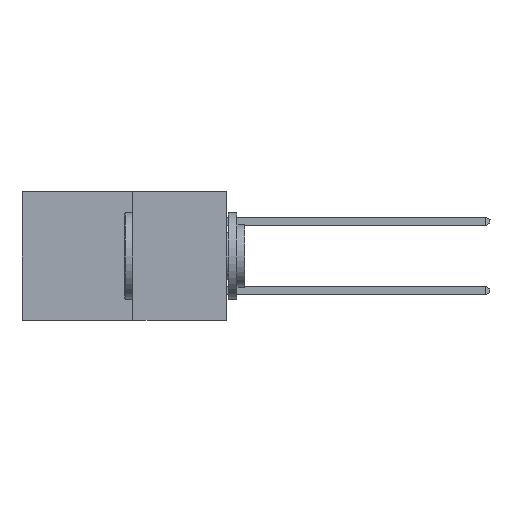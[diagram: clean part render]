
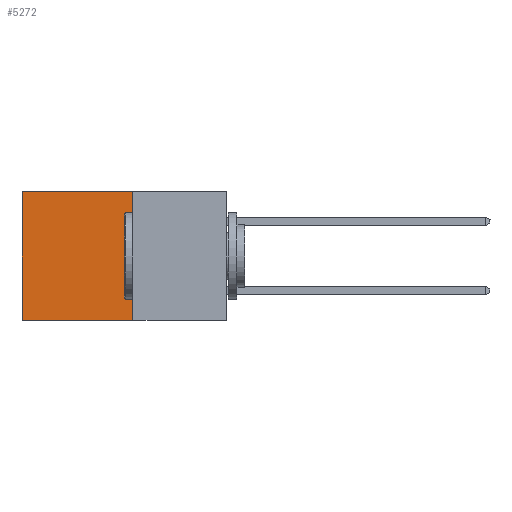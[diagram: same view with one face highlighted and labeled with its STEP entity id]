
A CAD part, left-side view. The second image highlights one B-rep face of the part: STEP entity #5272.
In plain terms, the highlighted planar face has unit normal (-1, 0, 0).
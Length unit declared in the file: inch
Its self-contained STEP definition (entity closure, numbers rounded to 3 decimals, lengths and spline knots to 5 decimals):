
#178 = CARTESIAN_POINT ( 'NONE',  ( 0.277, 0.59, -0.37 ) ) ;
#589 = EDGE_CURVE ( 'NONE', #18731, #17935, #16270, .T. ) ;
#727 = EDGE_LOOP ( 'NONE', ( #15447, #9353, #10430, #16326 ) ) ;
#1117 = CARTESIAN_POINT ( 'NONE',  ( 0.277, 0.27, -0.37 ) ) ;
#2031 = CARTESIAN_POINT ( 'NONE',  ( 0.277, 0.59, -0.37 ) ) ;
#2231 = CARTESIAN_POINT ( 'NONE',  ( 0.277, 0.59, 0. ) ) ;
#2304 = AXIS2_PLACEMENT_3D ( 'NONE', #13473, #13033, #13017 ) ;
#3314 = CARTESIAN_POINT ( 'NONE',  ( 0.277, 0.27, 0. ) ) ;
#3437 = CARTESIAN_POINT ( 'NONE',  ( 0.277, 0.27, -0.37 ) ) ;
#3535 = CARTESIAN_POINT ( 'NONE',  ( 0.277, 0.27, -0.37 ) ) ;
#5072 = DIRECTION ( 'NONE',  ( 0., 1., 0. ) ) ;
#5203 = DIRECTION ( 'NONE',  ( 0., 1., 0. ) ) ;
#5272 = ADVANCED_FACE ( 'NONE', ( #12234 ), #13311, .F. ) ;
#5304 = DIRECTION ( 'NONE',  ( 0., 0., -1. ) ) ;
#9308 = LINE ( 'NONE', #3314, #16820 ) ;
#9353 = ORIENTED_EDGE ( 'NONE', *, *, #19761, .F. ) ;
#9604 = VERTEX_POINT ( 'NONE', #20160 ) ;
#10359 = DIRECTION ( 'NONE',  ( 0., 0., -1. ) ) ;
#10430 = ORIENTED_EDGE ( 'NONE', *, *, #14724, .F. ) ;
#11042 = LINE ( 'NONE', #3437, #19675 ) ;
#11153 = LINE ( 'NONE', #3535, #19791 ) ;
#12234 = FACE_OUTER_BOUND ( 'NONE', #727, .T. ) ;
#13017 = DIRECTION ( 'NONE',  ( 0., 0., -1. ) ) ;
#13033 = DIRECTION ( 'NONE',  ( 1., 0., 0. ) ) ;
#13311 = PLANE ( 'NONE',  #2304 ) ;
#13473 = CARTESIAN_POINT ( 'NONE',  ( 0.277, 0.27, -0.37 ) ) ;
#14646 = EDGE_CURVE ( 'NONE', #9604, #18731, #9308, .T. ) ;
#14724 = EDGE_CURVE ( 'NONE', #9604, #15165, #11153, .T. ) ;
#15165 = VERTEX_POINT ( 'NONE', #1117 ) ;
#15447 = ORIENTED_EDGE ( 'NONE', *, *, #589, .T. ) ;
#16270 = LINE ( 'NONE', #178, #20857 ) ;
#16326 = ORIENTED_EDGE ( 'NONE', *, *, #14646, .T. ) ;
#16820 = VECTOR ( 'NONE', #5072, 39.37008 ) ;
#17935 = VERTEX_POINT ( 'NONE', #2031 ) ;
#18731 = VERTEX_POINT ( 'NONE', #2231 ) ;
#19675 = VECTOR ( 'NONE', #5203, 39.37008 ) ;
#19761 = EDGE_CURVE ( 'NONE', #15165, #17935, #11042, .T. ) ;
#19791 = VECTOR ( 'NONE', #5304, 39.37008 ) ;
#20160 = CARTESIAN_POINT ( 'NONE',  ( 0.277, 0.27, 0. ) ) ;
#20857 = VECTOR ( 'NONE', #10359, 39.37008 ) ;
